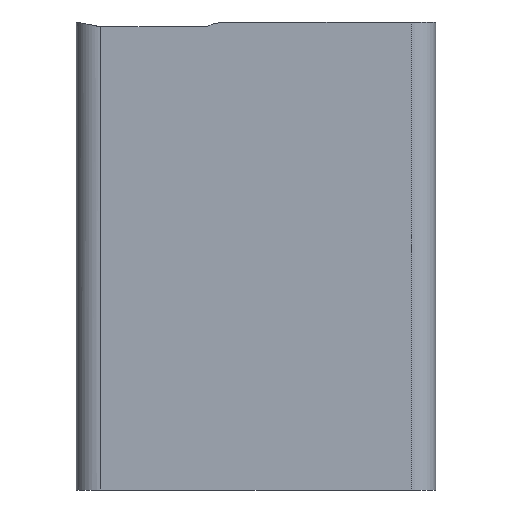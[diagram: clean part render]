
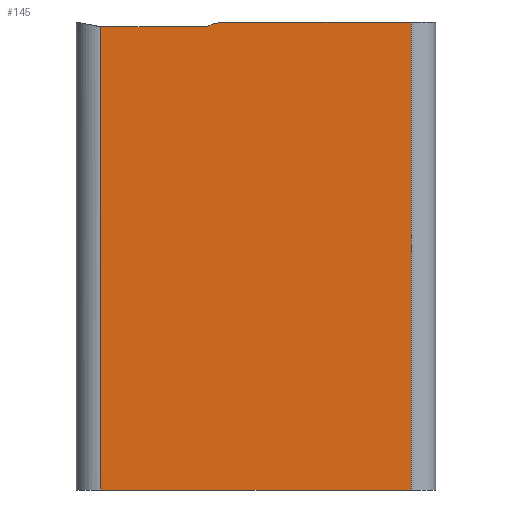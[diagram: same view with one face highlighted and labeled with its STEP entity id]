
A CAD part, left-side view. The second image highlights one B-rep face of the part: STEP entity #145.
In plain terms, the highlighted planar face has unit normal (-1, 0, 0).
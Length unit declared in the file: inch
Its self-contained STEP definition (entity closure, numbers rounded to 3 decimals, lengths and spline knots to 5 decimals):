
#1 = EDGE_LOOP ( 'NONE', ( #43, #479, #325, #546, #163, #430 ) ) ;
#19 = EDGE_CURVE ( 'NONE', #510, #266, #509, .T. ) ;
#26 = VERTEX_POINT ( 'NONE', #137 ) ;
#43 = ORIENTED_EDGE ( 'NONE', *, *, #92, .T. ) ;
#80 = AXIS2_PLACEMENT_3D ( 'NONE', #452, #506, #215 ) ;
#85 = DIRECTION ( 'NONE',  ( -1., 0., 0. ) ) ;
#92 = EDGE_CURVE ( 'NONE', #495, #588, #314, .T. ) ;
#105 = DIRECTION ( 'NONE',  ( 0., -1., 0. ) ) ;
#116 = CARTESIAN_POINT ( 'NONE',  ( -0.6, 0., 0.85 ) ) ;
#118 = VECTOR ( 'NONE', #554, 39.37008 ) ;
#119 = LINE ( 'NONE', #213, #631 ) ;
#129 = EDGE_CURVE ( 'NONE', #588, #460, #618, .T. ) ;
#130 = CARTESIAN_POINT ( 'NONE',  ( -0.6, 0.4243, 0.85 ) ) ;
#137 = CARTESIAN_POINT ( 'NONE',  ( -0.6, 0.68, 0.84 ) ) ;
#143 = CARTESIAN_POINT ( 'NONE',  ( -0.6, 0.05, -0.1 ) ) ;
#145 = ADVANCED_FACE ( 'NONE', ( #575 ), #605, .T. ) ;
#163 = ORIENTED_EDGE ( 'NONE', *, *, #568, .F. ) ;
#168 = VECTOR ( 'NONE', #566, 39.37008 ) ;
#188 = CARTESIAN_POINT ( 'NONE',  ( -0.6, 0., 0.84 ) ) ;
#190 = CARTESIAN_POINT ( 'NONE',  ( -0.6, 0.4243, 0.75 ) ) ;
#195 = EDGE_CURVE ( 'NONE', #26, #495, #119, .T. ) ;
#213 = CARTESIAN_POINT ( 'NONE',  ( -0.6, 0.68, 0. ) ) ;
#215 = DIRECTION ( 'NONE',  ( 0., 0., 1. ) ) ;
#235 = DIRECTION ( 'NONE',  ( 0., 0., 1. ) ) ;
#265 = VECTOR ( 'NONE', #344, 39.37008 ) ;
#266 = VERTEX_POINT ( 'NONE', #318 ) ;
#272 = EDGE_CURVE ( 'NONE', #510, #460, #455, .T. ) ;
#301 = CARTESIAN_POINT ( 'NONE',  ( -0.6, 0.05, 0. ) ) ;
#314 = LINE ( 'NONE', #647, #500 ) ;
#318 = CARTESIAN_POINT ( 'NONE',  ( -0.6, 0.46789, 0.84 ) ) ;
#324 = CARTESIAN_POINT ( 'NONE',  ( -0.6, 0.68, -0.1 ) ) ;
#325 = ORIENTED_EDGE ( 'NONE', *, *, #272, .F. ) ;
#333 = AXIS2_PLACEMENT_3D ( 'NONE', #190, #85, #235 ) ;
#344 = DIRECTION ( 'NONE',  ( 0., 0., 1. ) ) ;
#430 = ORIENTED_EDGE ( 'NONE', *, *, #195, .T. ) ;
#452 = CARTESIAN_POINT ( 'NONE',  ( -0.6, 0., 0. ) ) ;
#455 = LINE ( 'NONE', #116, #168 ) ;
#460 = VERTEX_POINT ( 'NONE', #533 ) ;
#479 = ORIENTED_EDGE ( 'NONE', *, *, #129, .T. ) ;
#495 = VERTEX_POINT ( 'NONE', #324 ) ;
#500 = VECTOR ( 'NONE', #105, 39.37008 ) ;
#506 = DIRECTION ( 'NONE',  ( -1., 0., 0. ) ) ;
#509 = CIRCLE ( 'NONE', #333, 0.1 ) ;
#510 = VERTEX_POINT ( 'NONE', #130 ) ;
#515 = LINE ( 'NONE', #188, #118 ) ;
#533 = CARTESIAN_POINT ( 'NONE',  ( -0.6, 0.05, 0.85 ) ) ;
#546 = ORIENTED_EDGE ( 'NONE', *, *, #19, .T. ) ;
#554 = DIRECTION ( 'NONE',  ( 0., -1., 0. ) ) ;
#566 = DIRECTION ( 'NONE',  ( 0., -1., 0. ) ) ;
#568 = EDGE_CURVE ( 'NONE', #26, #266, #515, .T. ) ;
#575 = FACE_OUTER_BOUND ( 'NONE', #1, .T. ) ;
#588 = VERTEX_POINT ( 'NONE', #143 ) ;
#605 = PLANE ( 'NONE',  #80 ) ;
#610 = DIRECTION ( 'NONE',  ( 0., 0., -1. ) ) ;
#618 = LINE ( 'NONE', #301, #265 ) ;
#631 = VECTOR ( 'NONE', #610, 39.37008 ) ;
#647 = CARTESIAN_POINT ( 'NONE',  ( -0.6, 0.73, -0.1 ) ) ;
